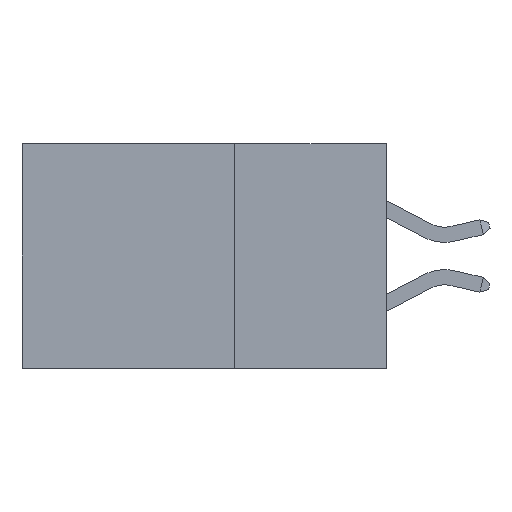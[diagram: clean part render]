
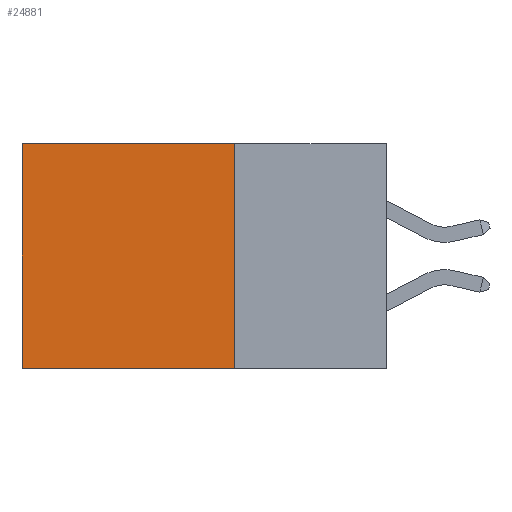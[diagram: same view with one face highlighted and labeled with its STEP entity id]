
A CAD part, left-side view. The second image highlights one B-rep face of the part: STEP entity #24881.
In plain terms, the highlighted planar face has unit normal (-1, 0, 0).
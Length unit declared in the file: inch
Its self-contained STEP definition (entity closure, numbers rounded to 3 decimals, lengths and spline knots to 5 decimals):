
#213 = LINE ( 'NONE', #14891, #16770 ) ;
#397 = DIRECTION ( 'NONE',  ( 0., 0., -1. ) ) ;
#404 = VERTEX_POINT ( 'NONE', #24361 ) ;
#498 = VERTEX_POINT ( 'NONE', #856 ) ;
#856 = CARTESIAN_POINT ( 'NONE',  ( 0.298, 0.6, 0. ) ) ;
#1162 = DIRECTION ( 'NONE',  ( 0., 0., -1. ) ) ;
#1964 = DIRECTION ( 'NONE',  ( 0., 1., 0. ) ) ;
#4003 = LINE ( 'NONE', #26913, #20407 ) ;
#6036 = VECTOR ( 'NONE', #397, 39.37008 ) ;
#6048 = DIRECTION ( 'NONE',  ( 0., 0., -1. ) ) ;
#7881 = DIRECTION ( 'NONE',  ( 0., 1., 0. ) ) ;
#9343 = ORIENTED_EDGE ( 'NONE', *, *, #22749, .T. ) ;
#9348 = VERTEX_POINT ( 'NONE', #26832 ) ;
#9500 = ORIENTED_EDGE ( 'NONE', *, *, #12740, .F. ) ;
#11356 = CARTESIAN_POINT ( 'NONE',  ( 0.298, 0.25, -0.37 ) ) ;
#11952 = CARTESIAN_POINT ( 'NONE',  ( 0.298, 0.25, 0. ) ) ;
#12740 = EDGE_CURVE ( 'NONE', #14083, #9348, #213, .T. ) ;
#14083 = VERTEX_POINT ( 'NONE', #11356 ) ;
#14096 = DIRECTION ( 'NONE',  ( 1., 0., 0. ) ) ;
#14740 = ORIENTED_EDGE ( 'NONE', *, *, #19679, .F. ) ;
#14891 = CARTESIAN_POINT ( 'NONE',  ( 0.298, 0.25, -0.37 ) ) ;
#15030 = VECTOR ( 'NONE', #6048, 39.37008 ) ;
#16770 = VECTOR ( 'NONE', #1964, 39.37008 ) ;
#17448 = LINE ( 'NONE', #17639, #6036 ) ;
#17639 = CARTESIAN_POINT ( 'NONE',  ( 0.298, 0.6, 0. ) ) ;
#18196 = EDGE_CURVE ( 'NONE', #404, #498, #4003, .T. ) ;
#19151 = EDGE_LOOP ( 'NONE', ( #9343, #9500, #14740, #23340 ) ) ;
#19679 = EDGE_CURVE ( 'NONE', #404, #14083, #20642, .T. ) ;
#20407 = VECTOR ( 'NONE', #7881, 39.37008 ) ;
#20642 = LINE ( 'NONE', #27204, #15030 ) ;
#22749 = EDGE_CURVE ( 'NONE', #498, #9348, #17448, .T. ) ;
#23340 = ORIENTED_EDGE ( 'NONE', *, *, #18196, .T. ) ;
#23601 = FACE_OUTER_BOUND ( 'NONE', #19151, .T. ) ;
#24361 = CARTESIAN_POINT ( 'NONE',  ( 0.298, 0.25, 0. ) ) ;
#24653 = PLANE ( 'NONE',  #27538 ) ;
#24881 = ADVANCED_FACE ( 'NONE', ( #23601 ), #24653, .F. ) ;
#26832 = CARTESIAN_POINT ( 'NONE',  ( 0.298, 0.6, -0.37 ) ) ;
#26913 = CARTESIAN_POINT ( 'NONE',  ( 0.298, 0.25, 0. ) ) ;
#27204 = CARTESIAN_POINT ( 'NONE',  ( 0.298, 0.25, 0. ) ) ;
#27538 = AXIS2_PLACEMENT_3D ( 'NONE', #11952, #14096, #1162 ) ;
